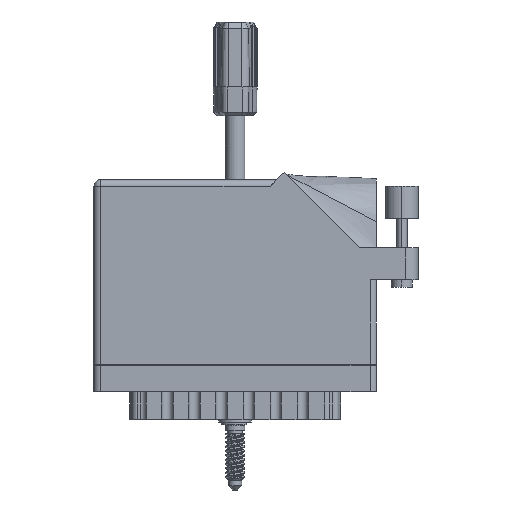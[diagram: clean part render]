
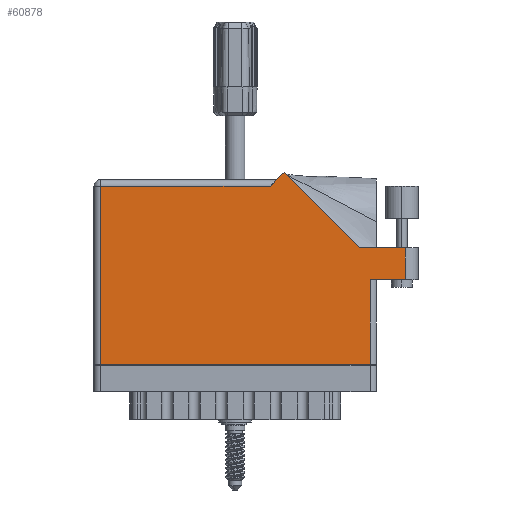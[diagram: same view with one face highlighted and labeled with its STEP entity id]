
A CAD part, front view. The second image highlights one B-rep face of the part: STEP entity #60878.
In plain terms, the highlighted face is planar.
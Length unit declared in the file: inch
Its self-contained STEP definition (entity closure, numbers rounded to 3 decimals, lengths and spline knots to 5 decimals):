
#580 = CARTESIAN_POINT ( 'NONE',  ( 2.993, 1.122, 0. ) ) ;
#2609 = LINE ( 'NONE', #32198, #67401 ) ;
#2682 = VERTEX_POINT ( 'NONE', #30345 ) ;
#3973 = VERTEX_POINT ( 'NONE', #66408 ) ;
#4668 = DIRECTION ( 'NONE',  ( -0.707, 0.707, 0. ) ) ;
#5839 = VECTOR ( 'NONE', #26617, 39.37008 ) ;
#6920 = CARTESIAN_POINT ( 'NONE',  ( 2.718, 0.815, 0. ) ) ;
#7213 = DIRECTION ( 'NONE',  ( 1., 0., 0. ) ) ;
#7967 = CARTESIAN_POINT ( 'NONE',  ( 0., 0., 0. ) ) ;
#10620 = PLANE ( 'NONE',  #74692 ) ;
#12226 = CARTESIAN_POINT ( 'NONE',  ( 0.062, 0., 0. ) ) ;
#13240 = DIRECTION ( 'NONE',  ( -1., 0., 0. ) ) ;
#14472 = DIRECTION ( 'NONE',  ( 1., 0., 0. ) ) ;
#16657 = DIRECTION ( 'NONE',  ( -1., 0., 0. ) ) ;
#17357 = CARTESIAN_POINT ( 'NONE',  ( 1.696, 1.713, 0. ) ) ;
#18266 = VECTOR ( 'NONE', #7213, 39.37008 ) ;
#18568 = EDGE_CURVE ( 'NONE', #79005, #19448, #23065, .T. ) ;
#19448 = VERTEX_POINT ( 'NONE', #17357 ) ;
#19883 = VERTEX_POINT ( 'NONE', #12226 ) ;
#20357 = ORIENTED_EDGE ( 'NONE', *, *, #37791, .T. ) ;
#20523 = ORIENTED_EDGE ( 'NONE', *, *, #72933, .T. ) ;
#20814 = CARTESIAN_POINT ( 'NONE',  ( 2.993, 0.815, 0. ) ) ;
#22827 = FACE_OUTER_BOUND ( 'NONE', #48799, .T. ) ;
#23065 = LINE ( 'NONE', #39626, #5839 ) ;
#23178 = EDGE_CURVE ( 'NONE', #3973, #34804, #58843, .T. ) ;
#23592 = CARTESIAN_POINT ( 'NONE',  ( 0.062, 1.713, 0. ) ) ;
#26617 = DIRECTION ( 'NONE',  ( -0.707, -0.707, 0. ) ) ;
#27007 = CARTESIAN_POINT ( 'NONE',  ( 2.55242, 1.122, 0. ) ) ;
#30345 = CARTESIAN_POINT ( 'NONE',  ( 2.656, 0., 0. ) ) ;
#30804 = VERTEX_POINT ( 'NONE', #580 ) ;
#32198 = CARTESIAN_POINT ( 'NONE',  ( 0., 1.713, 0. ) ) ;
#32699 = DIRECTION ( 'NONE',  ( 0., 1., 0. ) ) ;
#33569 = EDGE_CURVE ( 'NONE', #34804, #30804, #63811, .T. ) ;
#33978 = ORIENTED_EDGE ( 'NONE', *, *, #77608, .T. ) ;
#34804 = VERTEX_POINT ( 'NONE', #20814 ) ;
#35666 = DIRECTION ( 'NONE',  ( 0., 1., 0. ) ) ;
#37634 = EDGE_CURVE ( 'NONE', #52126, #79005, #68261, .T. ) ;
#37720 = VECTOR ( 'NONE', #16657, 39.37008 ) ;
#37791 = EDGE_CURVE ( 'NONE', #2682, #3973, #70244, .T. ) ;
#39626 = CARTESIAN_POINT ( 'NONE',  ( 1.758, 1.775, 0. ) ) ;
#39757 = LINE ( 'NONE', #67652, #37720 ) ;
#41334 = CARTESIAN_POINT ( 'NONE',  ( 2.993, 1.122, 0. ) ) ;
#41581 = ORIENTED_EDGE ( 'NONE', *, *, #80340, .T. ) ;
#41912 = ORIENTED_EDGE ( 'NONE', *, *, #23178, .T. ) ;
#41942 = VECTOR ( 'NONE', #4668, 39.37008 ) ;
#42867 = CARTESIAN_POINT ( 'NONE',  ( 0., 1.775, 0. ) ) ;
#43712 = LINE ( 'NONE', #7967, #57967 ) ;
#45850 = ORIENTED_EDGE ( 'NONE', *, *, #18568, .T. ) ;
#46904 = VECTOR ( 'NONE', #32699, 39.37008 ) ;
#48799 = EDGE_LOOP ( 'NONE', ( #41912, #79807, #41581, #78899, #45850, #33978, #66992, #20523, #20357 ) ) ;
#52126 = VERTEX_POINT ( 'NONE', #27007 ) ;
#52201 = DIRECTION ( 'NONE',  ( 0., -1., 0. ) ) ;
#52503 = CARTESIAN_POINT ( 'NONE',  ( 2.656, 0.815, 0. ) ) ;
#57967 = VECTOR ( 'NONE', #14472, 39.37008 ) ;
#58843 = LINE ( 'NONE', #6920, #18266 ) ;
#59392 = VECTOR ( 'NONE', #52201, 39.37008 ) ;
#60878 = ADVANCED_FACE ( 'NONE', ( #22827 ), #10620, .F. ) ;
#63811 = LINE ( 'NONE', #41334, #81051 ) ;
#66408 = CARTESIAN_POINT ( 'NONE',  ( 2.656, 0.815, 0. ) ) ;
#66814 = CARTESIAN_POINT ( 'NONE',  ( 1.82871, 1.84571, 0. ) ) ;
#66992 = ORIENTED_EDGE ( 'NONE', *, *, #70496, .T. ) ;
#67401 = VECTOR ( 'NONE', #13240, 39.37008 ) ;
#67652 = CARTESIAN_POINT ( 'NONE',  ( 3.118, 1.122, 0. ) ) ;
#67797 = DIRECTION ( 'NONE',  ( 0., 0., -1. ) ) ;
#68261 = LINE ( 'NONE', #82279, #41942 ) ;
#70244 = LINE ( 'NONE', #52503, #46904 ) ;
#70496 = EDGE_CURVE ( 'NONE', #76421, #19883, #76663, .T. ) ;
#72933 = EDGE_CURVE ( 'NONE', #19883, #2682, #43712, .T. ) ;
#74616 = DIRECTION ( 'NONE',  ( -1., 0., 0. ) ) ;
#74692 = AXIS2_PLACEMENT_3D ( 'NONE', #42867, #67797, #74616 ) ;
#76421 = VERTEX_POINT ( 'NONE', #23592 ) ;
#76663 = LINE ( 'NONE', #77473, #59392 ) ;
#77473 = CARTESIAN_POINT ( 'NONE',  ( 0.062, 0., 0. ) ) ;
#77608 = EDGE_CURVE ( 'NONE', #19448, #76421, #2609, .T. ) ;
#78899 = ORIENTED_EDGE ( 'NONE', *, *, #37634, .T. ) ;
#79005 = VERTEX_POINT ( 'NONE', #66814 ) ;
#79807 = ORIENTED_EDGE ( 'NONE', *, *, #33569, .T. ) ;
#80340 = EDGE_CURVE ( 'NONE', #30804, #52126, #39757, .T. ) ;
#81051 = VECTOR ( 'NONE', #35666, 39.37008 ) ;
#82279 = CARTESIAN_POINT ( 'NONE',  ( 2.55242, 1.122, 0. ) ) ;
